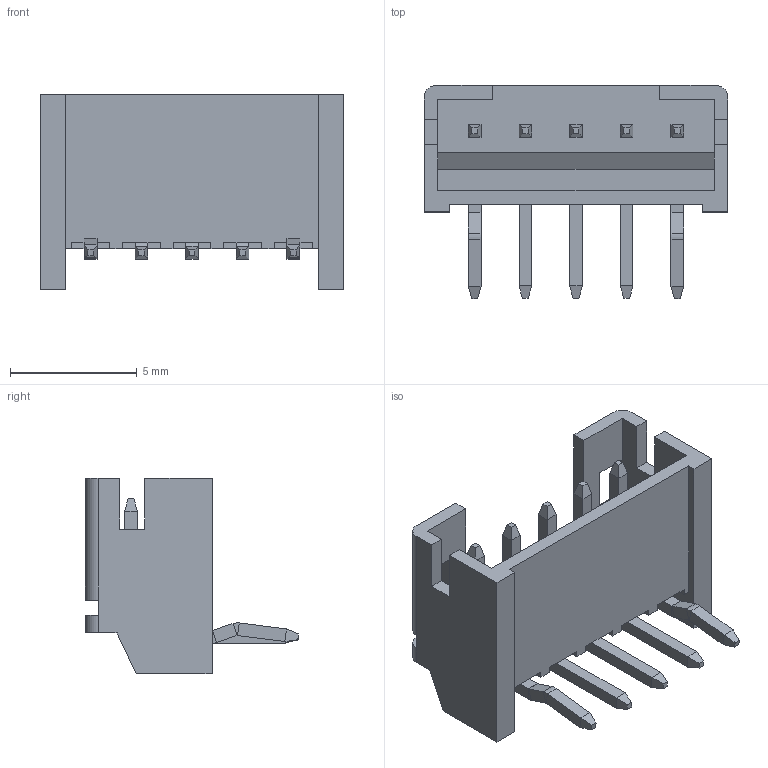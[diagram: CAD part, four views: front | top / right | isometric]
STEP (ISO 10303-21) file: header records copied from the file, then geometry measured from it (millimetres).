
FILE_DESCRIPTION (( 'STEP AP203' ), '1' );
FILE_NAME ('140-505-415-000.STEP', '2020-03-31T19:41:42', ( '' ), ( '' ), 'SwSTEP 2.0', 'SolidWorks 2016', '' );
FILE_SCHEMA (( 'CONFIG_CONTROL_DESIGN' ));
Length unit declared in the file: millimetre
Products named in the file (4): RA Housing_505; RA Contact_Str; 140-505-415-000; RA Contact_Kink
Assembly tree (6 placements, depth 2):
  140-505-415-000
    RA Housing_505
    RA Contact_Kink  x2
    RA Contact_Str  x3
Bounding box: 12 x 8.41 x 7.7 mm (x, y, z)
Volume: 159 mm3; surface area: 579.1 mm2
Topology: 6 solids, 6 shells, 229 faces, 541 edges, 322 vertices
Faces by surface type: plane 207, cylinder 22
Entity records: 4857 total; most frequent: CARTESIAN_POINT 767, ORIENTED_EDGE 754, DIRECTION 713, EDGE_CURVE 377, VECTOR 353, LINE 353, VERTEX_POINT 234, AXIS2_PLACEMENT_3D 180
